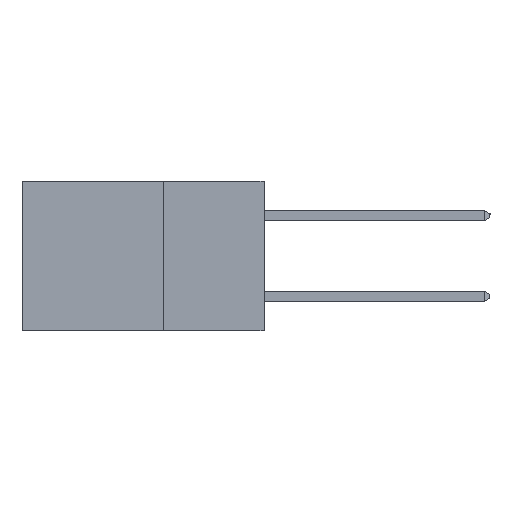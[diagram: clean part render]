
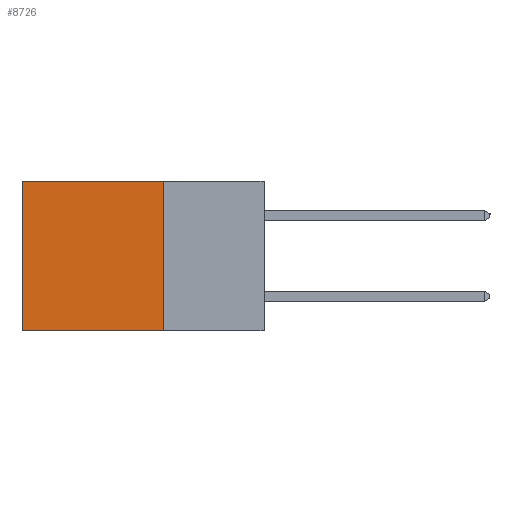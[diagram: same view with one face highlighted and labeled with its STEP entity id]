
A CAD part, left-side view. The second image highlights one B-rep face of the part: STEP entity #8726.
In plain terms, the highlighted planar face has unit normal (-1, 0, 0).
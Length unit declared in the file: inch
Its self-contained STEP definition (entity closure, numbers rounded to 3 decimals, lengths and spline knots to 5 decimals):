
#289 = LINE ( 'NONE', #7789, #2949 ) ;
#644 = VERTEX_POINT ( 'NONE', #2715 ) ;
#681 = LINE ( 'NONE', #6668, #9271 ) ;
#790 = PLANE ( 'NONE',  #9282 ) ;
#899 = CARTESIAN_POINT ( 'NONE',  ( 0.298, 0.25, 0. ) ) ;
#1003 = CARTESIAN_POINT ( 'NONE',  ( 0.298, 0.25, 0. ) ) ;
#1006 = DIRECTION ( 'NONE',  ( 1., 0., 0. ) ) ;
#1510 = EDGE_CURVE ( 'NONE', #13860, #9958, #289, .T. ) ;
#1545 = ORIENTED_EDGE ( 'NONE', *, *, #1510, .T. ) ;
#2052 = DIRECTION ( 'NONE',  ( 0., 1., 0. ) ) ;
#2114 = VECTOR ( 'NONE', #14218, 39.37008 ) ;
#2715 = CARTESIAN_POINT ( 'NONE',  ( 0.298, 0.25, -0.37 ) ) ;
#2949 = VECTOR ( 'NONE', #9123, 39.37008 ) ;
#3004 = DIRECTION ( 'NONE',  ( 0., 0., -1. ) ) ;
#3923 = ORIENTED_EDGE ( 'NONE', *, *, #6576, .F. ) ;
#4714 = CARTESIAN_POINT ( 'NONE',  ( 0.298, 0.6, -0.37 ) ) ;
#5701 = FACE_OUTER_BOUND ( 'NONE', #14284, .T. ) ;
#5840 = DIRECTION ( 'NONE',  ( 0., 0., -1. ) ) ;
#6447 = LINE ( 'NONE', #899, #8322 ) ;
#6576 = EDGE_CURVE ( 'NONE', #8634, #644, #681, .T. ) ;
#6668 = CARTESIAN_POINT ( 'NONE',  ( 0.298, 0.25, 0. ) ) ;
#7066 = CARTESIAN_POINT ( 'NONE',  ( 0.298, 0.6, 0. ) ) ;
#7429 = CARTESIAN_POINT ( 'NONE',  ( 0.298, 0.25, -0.37 ) ) ;
#7789 = CARTESIAN_POINT ( 'NONE',  ( 0.298, 0.6, 0. ) ) ;
#7973 = LINE ( 'NONE', #7429, #2114 ) ;
#8322 = VECTOR ( 'NONE', #2052, 39.37008 ) ;
#8634 = VERTEX_POINT ( 'NONE', #13286 ) ;
#8726 = ADVANCED_FACE ( 'NONE', ( #5701 ), #790, .F. ) ;
#9123 = DIRECTION ( 'NONE',  ( 0., 0., -1. ) ) ;
#9271 = VECTOR ( 'NONE', #3004, 39.37008 ) ;
#9282 = AXIS2_PLACEMENT_3D ( 'NONE', #1003, #1006, #5840 ) ;
#9958 = VERTEX_POINT ( 'NONE', #4714 ) ;
#10876 = ORIENTED_EDGE ( 'NONE', *, *, #12585, .T. ) ;
#11777 = ORIENTED_EDGE ( 'NONE', *, *, #14060, .F. ) ;
#12585 = EDGE_CURVE ( 'NONE', #8634, #13860, #6447, .T. ) ;
#13286 = CARTESIAN_POINT ( 'NONE',  ( 0.298, 0.25, 0. ) ) ;
#13860 = VERTEX_POINT ( 'NONE', #7066 ) ;
#14060 = EDGE_CURVE ( 'NONE', #644, #9958, #7973, .T. ) ;
#14218 = DIRECTION ( 'NONE',  ( 0., 1., 0. ) ) ;
#14284 = EDGE_LOOP ( 'NONE', ( #1545, #11777, #3923, #10876 ) ) ;
